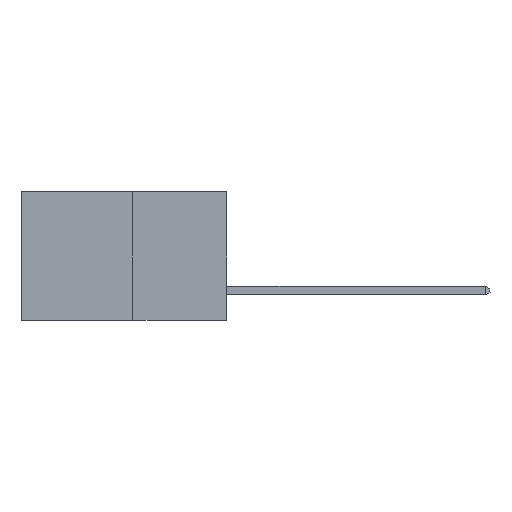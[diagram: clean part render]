
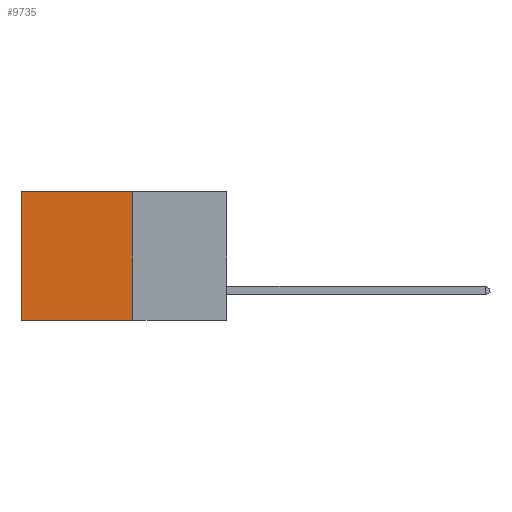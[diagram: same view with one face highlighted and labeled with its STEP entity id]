
A CAD part, left-side view. The second image highlights one B-rep face of the part: STEP entity #9735.
In plain terms, the highlighted planar face has unit normal (-1, 0, 0).
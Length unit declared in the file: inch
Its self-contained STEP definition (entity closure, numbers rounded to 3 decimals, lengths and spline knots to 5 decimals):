
#74 = DIRECTION ( 'NONE',  ( 1., 0., 0. ) ) ;
#974 = VECTOR ( 'NONE', #16902, 39.37008 ) ;
#1071 = LINE ( 'NONE', #19142, #17026 ) ;
#1281 = EDGE_LOOP ( 'NONE', ( #5463, #9854, #7108, #6156 ) ) ;
#1322 = VERTEX_POINT ( 'NONE', #9826 ) ;
#2373 = VERTEX_POINT ( 'NONE', #8004 ) ;
#3052 = PLANE ( 'NONE',  #6876 ) ;
#3388 = CARTESIAN_POINT ( 'NONE',  ( 0.277, 0.27, 0. ) ) ;
#3934 = EDGE_CURVE ( 'NONE', #1322, #18491, #1071, .T. ) ;
#5237 = EDGE_CURVE ( 'NONE', #2373, #18491, #6044, .T. ) ;
#5387 = VECTOR ( 'NONE', #8535, 39.37008 ) ;
#5463 = ORIENTED_EDGE ( 'NONE', *, *, #3934, .T. ) ;
#6044 = LINE ( 'NONE', #17081, #974 ) ;
#6156 = ORIENTED_EDGE ( 'NONE', *, *, #15781, .T. ) ;
#6537 = FACE_OUTER_BOUND ( 'NONE', #1281, .T. ) ;
#6643 = VERTEX_POINT ( 'NONE', #15660 ) ;
#6876 = AXIS2_PLACEMENT_3D ( 'NONE', #17959, #74, #10587 ) ;
#7082 = CARTESIAN_POINT ( 'NONE',  ( 0.277, 0.27, -0.37 ) ) ;
#7108 = ORIENTED_EDGE ( 'NONE', *, *, #16737, .F. ) ;
#8004 = CARTESIAN_POINT ( 'NONE',  ( 0.277, 0.27, -0.37 ) ) ;
#8535 = DIRECTION ( 'NONE',  ( 0., 0., -1. ) ) ;
#9735 = ADVANCED_FACE ( 'NONE', ( #6537 ), #3052, .F. ) ;
#9826 = CARTESIAN_POINT ( 'NONE',  ( 0.277, 0.59, 0. ) ) ;
#9854 = ORIENTED_EDGE ( 'NONE', *, *, #5237, .F. ) ;
#10587 = DIRECTION ( 'NONE',  ( 0., 0., -1. ) ) ;
#12349 = DIRECTION ( 'NONE',  ( 0., 1., 0. ) ) ;
#15660 = CARTESIAN_POINT ( 'NONE',  ( 0.277, 0.27, 0. ) ) ;
#15781 = EDGE_CURVE ( 'NONE', #6643, #1322, #17721, .T. ) ;
#16737 = EDGE_CURVE ( 'NONE', #6643, #2373, #17203, .T. ) ;
#16902 = DIRECTION ( 'NONE',  ( 0., 1., 0. ) ) ;
#17026 = VECTOR ( 'NONE', #18645, 39.37008 ) ;
#17081 = CARTESIAN_POINT ( 'NONE',  ( 0.277, 0.27, -0.37 ) ) ;
#17203 = LINE ( 'NONE', #7082, #5387 ) ;
#17721 = LINE ( 'NONE', #3388, #18168 ) ;
#17959 = CARTESIAN_POINT ( 'NONE',  ( 0.277, 0.27, -0.37 ) ) ;
#18168 = VECTOR ( 'NONE', #12349, 39.37008 ) ;
#18491 = VERTEX_POINT ( 'NONE', #18838 ) ;
#18645 = DIRECTION ( 'NONE',  ( 0., 0., -1. ) ) ;
#18838 = CARTESIAN_POINT ( 'NONE',  ( 0.277, 0.59, -0.37 ) ) ;
#19142 = CARTESIAN_POINT ( 'NONE',  ( 0.277, 0.59, -0.37 ) ) ;
